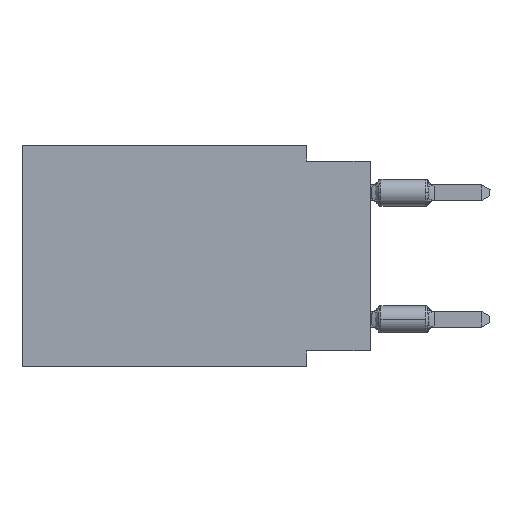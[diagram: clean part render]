
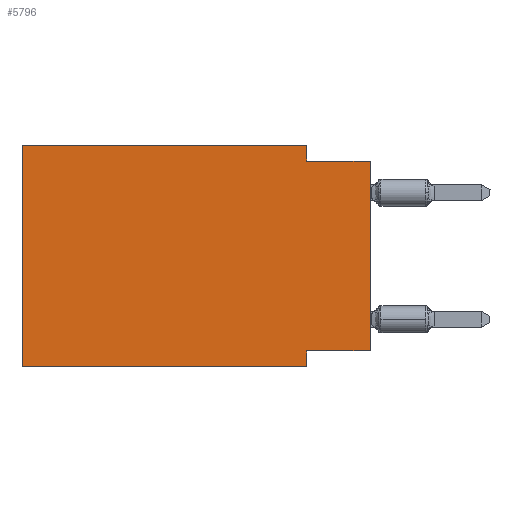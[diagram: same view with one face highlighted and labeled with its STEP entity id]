
A CAD part, left-side view. The second image highlights one B-rep face of the part: STEP entity #5796.
In plain terms, the highlighted planar face has unit normal (-1, 0, 0).
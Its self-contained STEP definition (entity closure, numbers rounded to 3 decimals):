
#3265 = VECTOR ( 'NONE', #32857, 1000. ) ;
#4776 = VECTOR ( 'NONE', #15175, 1000. ) ;
#5772 = DIRECTION ( 'NONE',  ( 0., 0., 1. ) ) ;
#5796 = ADVANCED_FACE ( 'NONE', ( #14076 ), #25721, .F. ) ;
#8220 = EDGE_CURVE ( 'NONE', #54788, #19337, #33358, .T. ) ;
#8260 = LINE ( 'NONE', #25353, #24448 ) ;
#10835 = DIRECTION ( 'NONE',  ( 0., -1., 0. ) ) ;
#11220 = DIRECTION ( 'NONE',  ( 0., 0., 1. ) ) ;
#11479 = CARTESIAN_POINT ( 'NONE',  ( 0., 2.54, -0.635 ) ) ;
#14076 = FACE_OUTER_BOUND ( 'NONE', #67539, .T. ) ;
#15175 = DIRECTION ( 'NONE',  ( 0., 0., -1. ) ) ;
#15310 = AXIS2_PLACEMENT_3D ( 'NONE', #63600, #35926, #69118 ) ;
#15907 = CARTESIAN_POINT ( 'NONE',  ( 0., 13.97, -8.89 ) ) ;
#15971 = LINE ( 'NONE', #55641, #23838 ) ;
#16223 = ORIENTED_EDGE ( 'NONE', *, *, #53108, .T. ) ;
#19337 = VERTEX_POINT ( 'NONE', #38326 ) ;
#23803 = VERTEX_POINT ( 'NONE', #31105 ) ;
#23838 = VECTOR ( 'NONE', #5772, 1000. ) ;
#24448 = VECTOR ( 'NONE', #35593, 1000. ) ;
#24453 = EDGE_CURVE ( 'NONE', #54788, #45131, #15971, .T. ) ;
#25353 = CARTESIAN_POINT ( 'NONE',  ( 0., 0., -8.255 ) ) ;
#25721 = PLANE ( 'NONE',  #15310 ) ;
#27261 = CARTESIAN_POINT ( 'NONE',  ( 0., 0., -8.255 ) ) ;
#28068 = DIRECTION ( 'NONE',  ( 0., -1., 0. ) ) ;
#29050 = LINE ( 'NONE', #50158, #40085 ) ;
#29400 = VERTEX_POINT ( 'NONE', #27261 ) ;
#31105 = CARTESIAN_POINT ( 'NONE',  ( 0., 0., -0.635 ) ) ;
#32857 = DIRECTION ( 'NONE',  ( 0., 0., -1. ) ) ;
#33358 = LINE ( 'NONE', #15907, #58525 ) ;
#34460 = CARTESIAN_POINT ( 'NONE',  ( 0., 0., -0.635 ) ) ;
#34788 = CARTESIAN_POINT ( 'NONE',  ( 0., 13.97, -8.89 ) ) ;
#34962 = ORIENTED_EDGE ( 'NONE', *, *, #45194, .F. ) ;
#35593 = DIRECTION ( 'NONE',  ( 0., 1., 0. ) ) ;
#35926 = DIRECTION ( 'NONE',  ( 1., 0., 0. ) ) ;
#38326 = CARTESIAN_POINT ( 'NONE',  ( 0., 2.54, -8.89 ) ) ;
#38708 = ORIENTED_EDGE ( 'NONE', *, *, #58241, .F. ) ;
#40085 = VECTOR ( 'NONE', #11220, 1000. ) ;
#42402 = VERTEX_POINT ( 'NONE', #68068 ) ;
#42572 = ORIENTED_EDGE ( 'NONE', *, *, #24453, .F. ) ;
#43211 = CARTESIAN_POINT ( 'NONE',  ( 0., 2.54, -8.89 ) ) ;
#44530 = VECTOR ( 'NONE', #10835, 1000. ) ;
#45131 = VERTEX_POINT ( 'NONE', #70775 ) ;
#45194 = EDGE_CURVE ( 'NONE', #42402, #53478, #64946, .T. ) ;
#48465 = ORIENTED_EDGE ( 'NONE', *, *, #54566, .F. ) ;
#48518 = ORIENTED_EDGE ( 'NONE', *, *, #62885, .F. ) ;
#50158 = CARTESIAN_POINT ( 'NONE',  ( 0., 0., 0. ) ) ;
#50482 = LINE ( 'NONE', #34460, #44530 ) ;
#51726 = LINE ( 'NONE', #68503, #55830 ) ;
#53108 = EDGE_CURVE ( 'NONE', #29400, #23803, #29050, .T. ) ;
#53478 = VERTEX_POINT ( 'NONE', #11479 ) ;
#54355 = CARTESIAN_POINT ( 'NONE',  ( 0., 2.54, 0. ) ) ;
#54566 = EDGE_CURVE ( 'NONE', #62021, #19337, #71627, .T. ) ;
#54788 = VERTEX_POINT ( 'NONE', #34788 ) ;
#55641 = CARTESIAN_POINT ( 'NONE',  ( 0., 13.97, 0. ) ) ;
#55830 = VECTOR ( 'NONE', #28068, 1000. ) ;
#58241 = EDGE_CURVE ( 'NONE', #53478, #23803, #50482, .T. ) ;
#58525 = VECTOR ( 'NONE', #66933, 1000. ) ;
#61017 = CARTESIAN_POINT ( 'NONE',  ( 0., 2.54, -8.255 ) ) ;
#61436 = ORIENTED_EDGE ( 'NONE', *, *, #8220, .T. ) ;
#61991 = ORIENTED_EDGE ( 'NONE', *, *, #68825, .F. ) ;
#62021 = VERTEX_POINT ( 'NONE', #61017 ) ;
#62885 = EDGE_CURVE ( 'NONE', #45131, #42402, #51726, .T. ) ;
#63600 = CARTESIAN_POINT ( 'NONE',  ( 0., 13.97, 0. ) ) ;
#64946 = LINE ( 'NONE', #54355, #3265 ) ;
#66933 = DIRECTION ( 'NONE',  ( 0., -1., 0. ) ) ;
#67539 = EDGE_LOOP ( 'NONE', ( #16223, #38708, #34962, #48518, #42572, #61436, #48465, #61991 ) ) ;
#68068 = CARTESIAN_POINT ( 'NONE',  ( 0., 2.54, 0. ) ) ;
#68503 = CARTESIAN_POINT ( 'NONE',  ( 0., 13.97, 0. ) ) ;
#68825 = EDGE_CURVE ( 'NONE', #29400, #62021, #8260, .T. ) ;
#69118 = DIRECTION ( 'NONE',  ( 0., 0., -1. ) ) ;
#70775 = CARTESIAN_POINT ( 'NONE',  ( 0., 13.97, 0. ) ) ;
#71627 = LINE ( 'NONE', #43211, #4776 ) ;
